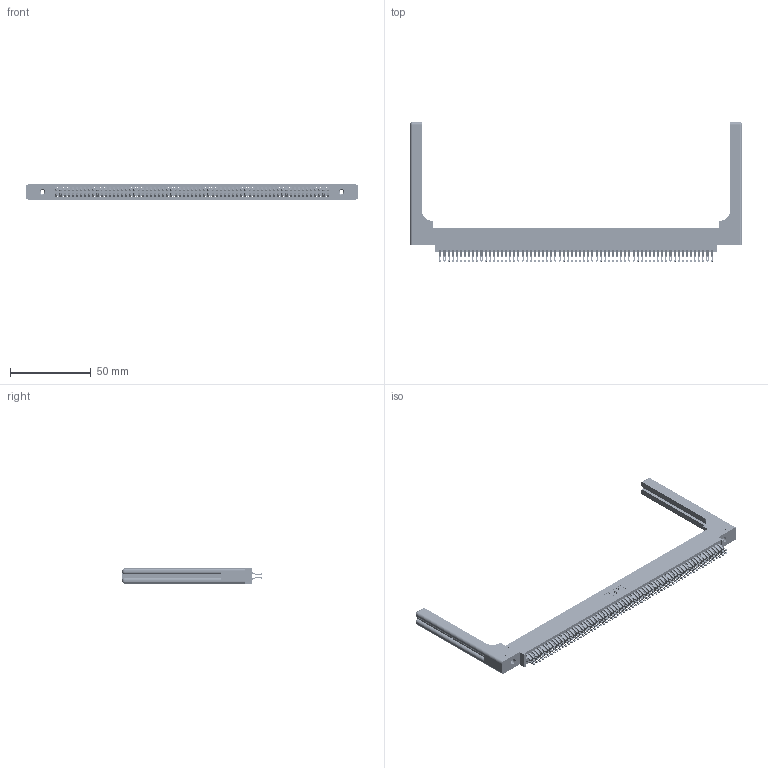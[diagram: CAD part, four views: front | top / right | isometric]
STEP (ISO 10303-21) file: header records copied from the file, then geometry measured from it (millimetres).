
FILE_DESCRIPTION (( 'STEP AP203' ), '1' );
FILE_NAME ('345-134-555-858.STEP', '2019-11-08T03:54:28', ( '' ), ( '' ), 'SwSTEP 2.0', 'SolidWorks 2016', '' );
FILE_SCHEMA (( 'CONFIG_CONTROL_DESIGN' ));
Length unit declared in the file: inch
Products named in the file (5): 345-292-001_555 Tail; 345-250-001_345-250-001-102; 345-134-555-858; 345-220-058_345-220-058; 345 Part_0.170 Offset - 0.156 Dia-TH
Assembly tree (139 placements, depth 2):
  345-134-555-858
    345 Part_0.170 Offset - 0.156 Dia-TH
    345-292-001_555 Tail  x134
    345-250-001_345-250-001-102  x2
    345-220-058_345-220-058  x2
Bounding box: 205.21 x 86.41 x 9.4 mm (x, y, z)
Volume: 28916.4 mm3; surface area: 37254.1 mm2
Topology: 139 solids, 139 shells, 7890 faces, 24737 edges, 16470 vertices
Faces by surface type: plane 4386, cylinder 3444, bspline 36, cone 12, sphere 8, torus 4
Entity records: 54844 total; most frequent: CARTESIAN_POINT 10199, ORIENTED_EDGE 8900, DIRECTION 7862, EDGE_CURVE 4450, LINE 3938, VECTOR 3938, VERTEX_POINT 2958, AXIS2_PLACEMENT_3D 1962
